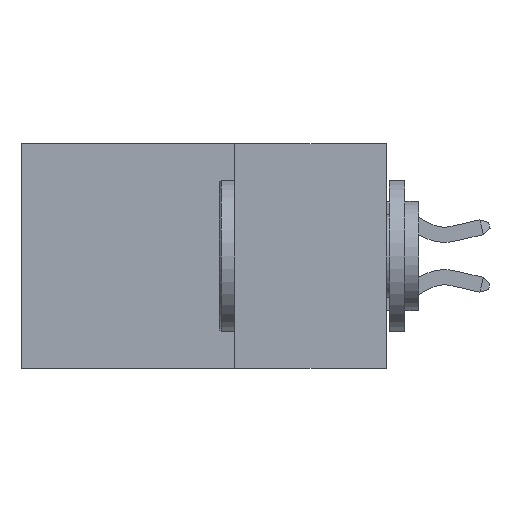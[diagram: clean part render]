
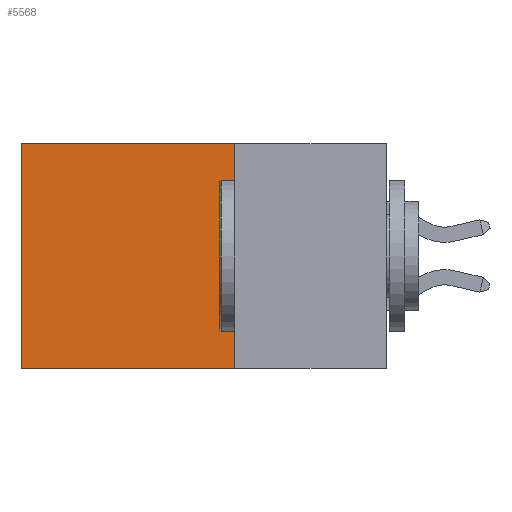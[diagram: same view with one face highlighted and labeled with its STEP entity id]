
A CAD part, left-side view. The second image highlights one B-rep face of the part: STEP entity #5568.
In plain terms, the highlighted planar face has unit normal (-1, 0, 0).
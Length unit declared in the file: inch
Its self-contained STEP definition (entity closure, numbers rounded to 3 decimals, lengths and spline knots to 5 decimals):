
#475 = CARTESIAN_POINT ( 'NONE',  ( 0.2615, 0.25, -0.37 ) ) ;
#711 = VECTOR ( 'NONE', #6448, 39.37008 ) ;
#1501 = ORIENTED_EDGE ( 'NONE', *, *, #10340, .F. ) ;
#3658 = CARTESIAN_POINT ( 'NONE',  ( 0.2615, 0.25, 0. ) ) ;
#3755 = ORIENTED_EDGE ( 'NONE', *, *, #12761, .T. ) ;
#5491 = DIRECTION ( 'NONE',  ( 0., 1., 0. ) ) ;
#5568 = ADVANCED_FACE ( 'NONE', ( #15063 ), #10899, .F. ) ;
#5758 = CARTESIAN_POINT ( 'NONE',  ( 0.2615, 0.25, -0.37 ) ) ;
#6158 = DIRECTION ( 'NONE',  ( 0., 0., -1. ) ) ;
#6448 = DIRECTION ( 'NONE',  ( 0., 1., 0. ) ) ;
#6841 = LINE ( 'NONE', #16074, #12514 ) ;
#7184 = VERTEX_POINT ( 'NONE', #7630 ) ;
#7372 = EDGE_LOOP ( 'NONE', ( #15587, #17039, #1501, #3755 ) ) ;
#7630 = CARTESIAN_POINT ( 'NONE',  ( 0.2615, 0.6, -0.37 ) ) ;
#7950 = CARTESIAN_POINT ( 'NONE',  ( 0.2615, 0.25, -0.37 ) ) ;
#8534 = VERTEX_POINT ( 'NONE', #7950 ) ;
#8976 = LINE ( 'NONE', #16408, #10404 ) ;
#9104 = LINE ( 'NONE', #3658, #711 ) ;
#9822 = DIRECTION ( 'NONE',  ( 0., 0., -1. ) ) ;
#10316 = CARTESIAN_POINT ( 'NONE',  ( 0.2615, 0.25, 0. ) ) ;
#10340 = EDGE_CURVE ( 'NONE', #15459, #8534, #15738, .T. ) ;
#10404 = VECTOR ( 'NONE', #12474, 39.37008 ) ;
#10899 = PLANE ( 'NONE',  #13558 ) ;
#11497 = EDGE_CURVE ( 'NONE', #15894, #7184, #8976, .T. ) ;
#12474 = DIRECTION ( 'NONE',  ( 0., 0., -1. ) ) ;
#12514 = VECTOR ( 'NONE', #5491, 39.37008 ) ;
#12761 = EDGE_CURVE ( 'NONE', #15459, #15894, #9104, .T. ) ;
#13558 = AXIS2_PLACEMENT_3D ( 'NONE', #5758, #16594, #9822 ) ;
#13763 = VECTOR ( 'NONE', #6158, 39.37008 ) ;
#15063 = FACE_OUTER_BOUND ( 'NONE', #7372, .T. ) ;
#15459 = VERTEX_POINT ( 'NONE', #10316 ) ;
#15587 = ORIENTED_EDGE ( 'NONE', *, *, #11497, .T. ) ;
#15738 = LINE ( 'NONE', #475, #13763 ) ;
#15894 = VERTEX_POINT ( 'NONE', #15986 ) ;
#15986 = CARTESIAN_POINT ( 'NONE',  ( 0.2615, 0.6, 0. ) ) ;
#16074 = CARTESIAN_POINT ( 'NONE',  ( 0.2615, 0.25, -0.37 ) ) ;
#16107 = EDGE_CURVE ( 'NONE', #8534, #7184, #6841, .T. ) ;
#16408 = CARTESIAN_POINT ( 'NONE',  ( 0.2615, 0.6, -0.37 ) ) ;
#16594 = DIRECTION ( 'NONE',  ( 1., 0., 0. ) ) ;
#17039 = ORIENTED_EDGE ( 'NONE', *, *, #16107, .F. ) ;
